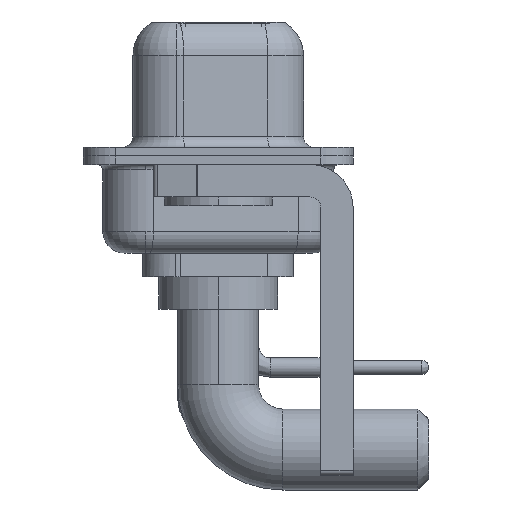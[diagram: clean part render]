
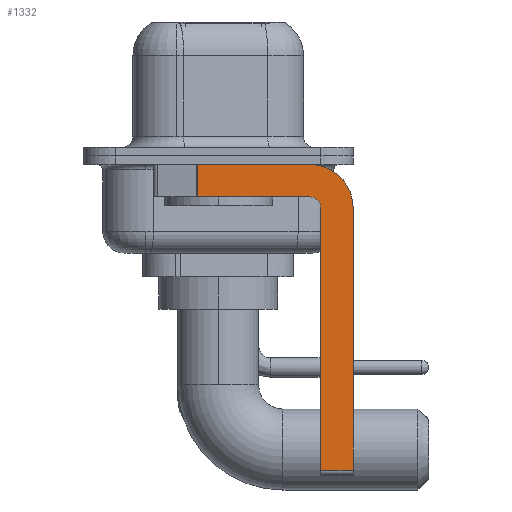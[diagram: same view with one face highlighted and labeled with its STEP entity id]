
A CAD part, left-side view. The second image highlights one B-rep face of the part: STEP entity #1332.
In plain terms, the highlighted planar face has unit normal (-1, 0, 0).
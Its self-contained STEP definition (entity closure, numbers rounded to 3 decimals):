
#81 = ORIENTED_EDGE ( 'NONE', *, *, #11160, .T. ) ;
#489 = CARTESIAN_POINT ( 'NONE',  ( -2.9, -4.25, -0.4 ) ) ;
#1161 = VECTOR ( 'NONE', #1947, 1000. ) ;
#1245 = CARTESIAN_POINT ( 'NONE',  ( -2.9, 0.978, -1.9 ) ) ;
#1332 = ADVANCED_FACE ( 'NONE', ( #19974 ), #13390, .F. ) ;
#1479 = DIRECTION ( 'NONE',  ( 0., 0., 1. ) ) ;
#1594 = VECTOR ( 'NONE', #13513, 1000. ) ;
#1714 = CARTESIAN_POINT ( 'NONE',  ( -2.9, -6.25, -2.4 ) ) ;
#1947 = DIRECTION ( 'NONE',  ( 0., 1., 0. ) ) ;
#2027 = EDGE_LOOP ( 'NONE', ( #14012, #81, #12059, #3822, #13817, #20184, #15656, #16714 ) ) ;
#2170 = CARTESIAN_POINT ( 'NONE',  ( -2.9, 0.978, -1.9 ) ) ;
#2203 = EDGE_CURVE ( 'NONE', #9605, #12621, #6937, .T. ) ;
#2262 = LINE ( 'NONE', #13844, #1594 ) ;
#2270 = LINE ( 'NONE', #10238, #1161 ) ;
#2554 = VECTOR ( 'NONE', #19507, 1000. ) ;
#3303 = CARTESIAN_POINT ( 'NONE',  ( -2.9, -4.25, -1.9 ) ) ;
#3822 = ORIENTED_EDGE ( 'NONE', *, *, #15134, .F. ) ;
#4318 = VERTEX_POINT ( 'NONE', #17040 ) ;
#4955 = DIRECTION ( 'NONE',  ( 0., 0., -1. ) ) ;
#5065 = DIRECTION ( 'NONE',  ( 1., 0., 0. ) ) ;
#5103 = DIRECTION ( 'NONE',  ( 1., 0., 0. ) ) ;
#6163 = CIRCLE ( 'NONE', #18419, 0.5 ) ;
#6844 = CARTESIAN_POINT ( 'NONE',  ( -2.9, -4.25, -2.4 ) ) ;
#6937 = CIRCLE ( 'NONE', #10063, 2. ) ;
#7302 = DIRECTION ( 'NONE',  ( 0., 0., -1. ) ) ;
#7604 = VERTEX_POINT ( 'NONE', #8136 ) ;
#8136 = CARTESIAN_POINT ( 'NONE',  ( -2.9, -4.75, -2.4 ) ) ;
#8253 = LINE ( 'NONE', #9768, #11587 ) ;
#8321 = DIRECTION ( 'NONE',  ( 0., -1., 0. ) ) ;
#8404 = CARTESIAN_POINT ( 'NONE',  ( -2.9, -4.25, -2.4 ) ) ;
#8431 = LINE ( 'NONE', #15104, #17983 ) ;
#8489 = CARTESIAN_POINT ( 'NONE',  ( -2.9, -6.25, -14.55 ) ) ;
#9572 = CARTESIAN_POINT ( 'NONE',  ( -2.9, -6.25, -2.4 ) ) ;
#9605 = VERTEX_POINT ( 'NONE', #489 ) ;
#9768 = CARTESIAN_POINT ( 'NONE',  ( -2.9, -4.75, -14.8 ) ) ;
#10063 = AXIS2_PLACEMENT_3D ( 'NONE', #20052, #5065, #4955 ) ;
#10238 = CARTESIAN_POINT ( 'NONE',  ( -2.9, -4.25, -1.9 ) ) ;
#10261 = EDGE_CURVE ( 'NONE', #12621, #11692, #16699, .T. ) ;
#10461 = DIRECTION ( 'NONE',  ( 0., 0., 1. ) ) ;
#11160 = EDGE_CURVE ( 'NONE', #4318, #17900, #15192, .T. ) ;
#11587 = VECTOR ( 'NONE', #1479, 1000. ) ;
#11692 = VERTEX_POINT ( 'NONE', #8489 ) ;
#12059 = ORIENTED_EDGE ( 'NONE', *, *, #20349, .F. ) ;
#12544 = VERTEX_POINT ( 'NONE', #3303 ) ;
#12621 = VERTEX_POINT ( 'NONE', #9572 ) ;
#12917 = EDGE_CURVE ( 'NONE', #19079, #11692, #2262, .T. ) ;
#13390 = PLANE ( 'NONE',  #13880 ) ;
#13503 = DIRECTION ( 'NONE',  ( 0., 0., -1. ) ) ;
#13513 = DIRECTION ( 'NONE',  ( 0., -1., 0. ) ) ;
#13817 = ORIENTED_EDGE ( 'NONE', *, *, #19324, .F. ) ;
#13844 = CARTESIAN_POINT ( 'NONE',  ( -2.9, -4.25, -14.55 ) ) ;
#13880 = AXIS2_PLACEMENT_3D ( 'NONE', #6844, #5103, #13503 ) ;
#14012 = ORIENTED_EDGE ( 'NONE', *, *, #19736, .F. ) ;
#15104 = CARTESIAN_POINT ( 'NONE',  ( -2.9, 3., -0.4 ) ) ;
#15134 = EDGE_CURVE ( 'NONE', #7604, #12544, #6163, .T. ) ;
#15192 = LINE ( 'NONE', #2170, #17284 ) ;
#15656 = ORIENTED_EDGE ( 'NONE', *, *, #10261, .F. ) ;
#16699 = LINE ( 'NONE', #1714, #2554 ) ;
#16714 = ORIENTED_EDGE ( 'NONE', *, *, #2203, .F. ) ;
#17040 = CARTESIAN_POINT ( 'NONE',  ( -2.9, 0.978, -0.4 ) ) ;
#17178 = DIRECTION ( 'NONE',  ( -1., 0., 0. ) ) ;
#17284 = VECTOR ( 'NONE', #7302, 1000. ) ;
#17900 = VERTEX_POINT ( 'NONE', #1245 ) ;
#17983 = VECTOR ( 'NONE', #8321, 1000. ) ;
#18419 = AXIS2_PLACEMENT_3D ( 'NONE', #8404, #17178, #10461 ) ;
#19079 = VERTEX_POINT ( 'NONE', #21177 ) ;
#19324 = EDGE_CURVE ( 'NONE', #19079, #7604, #8253, .T. ) ;
#19507 = DIRECTION ( 'NONE',  ( 0., 0., -1. ) ) ;
#19736 = EDGE_CURVE ( 'NONE', #4318, #9605, #8431, .T. ) ;
#19974 = FACE_OUTER_BOUND ( 'NONE', #2027, .T. ) ;
#20052 = CARTESIAN_POINT ( 'NONE',  ( -2.9, -4.25, -2.4 ) ) ;
#20184 = ORIENTED_EDGE ( 'NONE', *, *, #12917, .T. ) ;
#20349 = EDGE_CURVE ( 'NONE', #12544, #17900, #2270, .T. ) ;
#21177 = CARTESIAN_POINT ( 'NONE',  ( -2.9, -4.75, -14.55 ) ) ;
